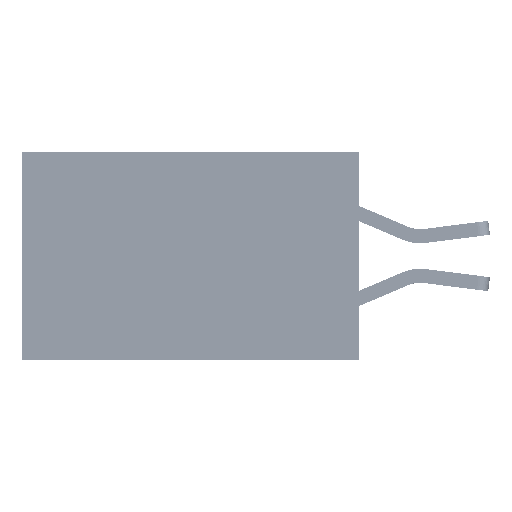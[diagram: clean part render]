
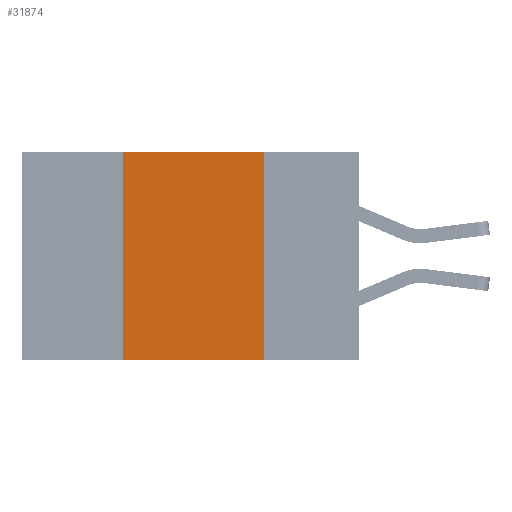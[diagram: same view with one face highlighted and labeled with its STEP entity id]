
A CAD part, left-side view. The second image highlights one B-rep face of the part: STEP entity #31874.
In plain terms, the highlighted planar face has unit normal (-1, 0, 0).
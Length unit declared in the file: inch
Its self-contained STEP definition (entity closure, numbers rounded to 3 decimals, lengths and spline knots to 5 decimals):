
#696 = PLANE ( 'NONE',  #6028 ) ;
#1235 = VERTEX_POINT ( 'NONE', #15381 ) ;
#3406 = ORIENTED_EDGE ( 'NONE', *, *, #41574, .F. ) ;
#3493 = DIRECTION ( 'NONE',  ( 0., -1., 0. ) ) ;
#5620 = VERTEX_POINT ( 'NONE', #34719 ) ;
#6028 = AXIS2_PLACEMENT_3D ( 'NONE', #10137, #16793, #16582 ) ;
#7059 = ORIENTED_EDGE ( 'NONE', *, *, #27084, .F. ) ;
#8269 = VECTOR ( 'NONE', #39379, 39.37008 ) ;
#10137 = CARTESIAN_POINT ( 'NONE',  ( 0., 0.6, 0. ) ) ;
#10200 = EDGE_LOOP ( 'NONE', ( #7059, #3406, #12104, #27075 ) ) ;
#12104 = ORIENTED_EDGE ( 'NONE', *, *, #12661, .F. ) ;
#12661 = EDGE_CURVE ( 'NONE', #5620, #36957, #22490, .T. ) ;
#12718 = VECTOR ( 'NONE', #36785, 39.37008 ) ;
#13353 = FACE_OUTER_BOUND ( 'NONE', #10200, .T. ) ;
#13778 = LINE ( 'NONE', #36880, #22750 ) ;
#15381 = CARTESIAN_POINT ( 'NONE',  ( 0., 0.17, 0. ) ) ;
#16582 = DIRECTION ( 'NONE',  ( 0., 0., -1. ) ) ;
#16793 = DIRECTION ( 'NONE',  ( 1., 0., 0. ) ) ;
#19902 = CARTESIAN_POINT ( 'NONE',  ( 0., 0.6, -0.37 ) ) ;
#21424 = VECTOR ( 'NONE', #25926, 39.37008 ) ;
#22490 = LINE ( 'NONE', #35545, #21424 ) ;
#22750 = VECTOR ( 'NONE', #3493, 39.37008 ) ;
#23742 = CARTESIAN_POINT ( 'NONE',  ( 0., 0.17, 0. ) ) ;
#25926 = DIRECTION ( 'NONE',  ( 0., 0., 1. ) ) ;
#26325 = LINE ( 'NONE', #23742, #12718 ) ;
#27075 = ORIENTED_EDGE ( 'NONE', *, *, #36749, .T. ) ;
#27084 = EDGE_CURVE ( 'NONE', #1235, #35783, #26325, .T. ) ;
#29221 = CARTESIAN_POINT ( 'NONE',  ( 0., 0.17, -0.37 ) ) ;
#31874 = ADVANCED_FACE ( 'NONE', ( #13353 ), #696, .F. ) ;
#32740 = LINE ( 'NONE', #19902, #8269 ) ;
#33163 = CARTESIAN_POINT ( 'NONE',  ( 0., 0.42, 0. ) ) ;
#34719 = CARTESIAN_POINT ( 'NONE',  ( 0., 0.42, -0.37 ) ) ;
#35545 = CARTESIAN_POINT ( 'NONE',  ( 0., 0.42, 0. ) ) ;
#35783 = VERTEX_POINT ( 'NONE', #29221 ) ;
#36749 = EDGE_CURVE ( 'NONE', #5620, #35783, #32740, .T. ) ;
#36785 = DIRECTION ( 'NONE',  ( 0., 0., -1. ) ) ;
#36880 = CARTESIAN_POINT ( 'NONE',  ( 0., 0.6, 0. ) ) ;
#36957 = VERTEX_POINT ( 'NONE', #33163 ) ;
#39379 = DIRECTION ( 'NONE',  ( 0., -1., 0. ) ) ;
#41574 = EDGE_CURVE ( 'NONE', #36957, #1235, #13778, .T. ) ;
